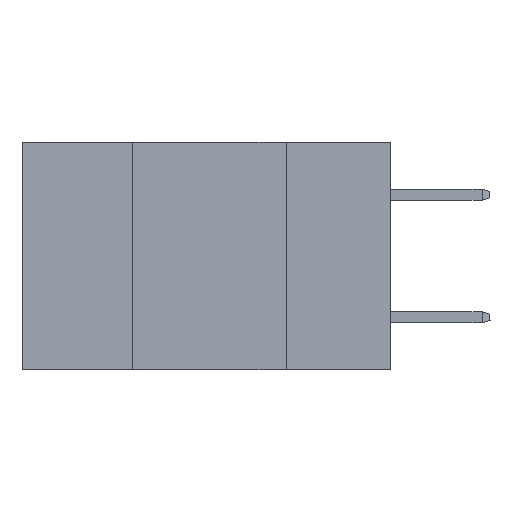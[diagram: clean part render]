
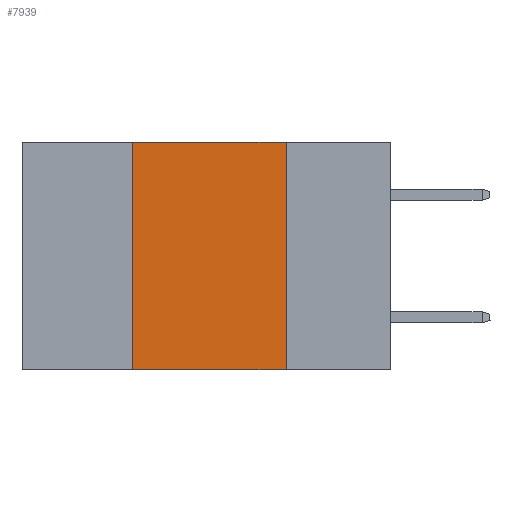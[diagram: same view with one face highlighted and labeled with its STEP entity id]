
A CAD part, left-side view. The second image highlights one B-rep face of the part: STEP entity #7939.
In plain terms, the highlighted planar face has unit normal (-1, 0, 0).
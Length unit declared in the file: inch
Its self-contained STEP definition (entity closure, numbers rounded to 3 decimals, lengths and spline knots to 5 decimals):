
#281 = LINE ( 'NONE', #3648, #5363 ) ;
#696 = EDGE_CURVE ( 'NONE', #11464, #17121, #1826, .T. ) ;
#832 = EDGE_LOOP ( 'NONE', ( #17126, #20765, #9822, #13039 ) ) ;
#1763 = DIRECTION ( 'NONE',  ( 0., 0., 1. ) ) ;
#1826 = LINE ( 'NONE', #14221, #5634 ) ;
#2089 = DIRECTION ( 'NONE',  ( 0., 0., -1. ) ) ;
#2645 = CARTESIAN_POINT ( 'NONE',  ( 0., 0.17, 0. ) ) ;
#3424 = EDGE_CURVE ( 'NONE', #17121, #15181, #281, .T. ) ;
#3464 = CARTESIAN_POINT ( 'NONE',  ( 0., 0.42, 0. ) ) ;
#3470 = CARTESIAN_POINT ( 'NONE',  ( 0., 0.6, 0. ) ) ;
#3648 = CARTESIAN_POINT ( 'NONE',  ( 0., 0.17, 0. ) ) ;
#5363 = VECTOR ( 'NONE', #2089, 39.37008 ) ;
#5634 = VECTOR ( 'NONE', #9278, 39.37008 ) ;
#6985 = PLANE ( 'NONE',  #19866 ) ;
#7691 = CARTESIAN_POINT ( 'NONE',  ( 0., 0.6, -0.37 ) ) ;
#7939 = ADVANCED_FACE ( 'NONE', ( #20541 ), #6985, .F. ) ;
#8173 = CARTESIAN_POINT ( 'NONE',  ( 0., 0.17, -0.37 ) ) ;
#8841 = VECTOR ( 'NONE', #1763, 39.37008 ) ;
#9220 = DIRECTION ( 'NONE',  ( 0., -1., 0. ) ) ;
#9278 = DIRECTION ( 'NONE',  ( 0., -1., 0. ) ) ;
#9508 = EDGE_CURVE ( 'NONE', #11034, #15181, #20712, .T. ) ;
#9822 = ORIENTED_EDGE ( 'NONE', *, *, #20562, .F. ) ;
#10259 = DIRECTION ( 'NONE',  ( 0., 0., -1. ) ) ;
#10483 = CARTESIAN_POINT ( 'NONE',  ( 0., 0.42, -0.37 ) ) ;
#11034 = VERTEX_POINT ( 'NONE', #10483 ) ;
#11436 = DIRECTION ( 'NONE',  ( 1., 0., 0. ) ) ;
#11464 = VERTEX_POINT ( 'NONE', #20120 ) ;
#13039 = ORIENTED_EDGE ( 'NONE', *, *, #9508, .T. ) ;
#13930 = VECTOR ( 'NONE', #9220, 39.37008 ) ;
#14221 = CARTESIAN_POINT ( 'NONE',  ( 0., 0.6, 0. ) ) ;
#15181 = VERTEX_POINT ( 'NONE', #8173 ) ;
#17121 = VERTEX_POINT ( 'NONE', #2645 ) ;
#17126 = ORIENTED_EDGE ( 'NONE', *, *, #3424, .F. ) ;
#17413 = LINE ( 'NONE', #3464, #8841 ) ;
#19866 = AXIS2_PLACEMENT_3D ( 'NONE', #3470, #11436, #10259 ) ;
#20120 = CARTESIAN_POINT ( 'NONE',  ( 0., 0.42, 0. ) ) ;
#20541 = FACE_OUTER_BOUND ( 'NONE', #832, .T. ) ;
#20562 = EDGE_CURVE ( 'NONE', #11034, #11464, #17413, .T. ) ;
#20712 = LINE ( 'NONE', #7691, #13930 ) ;
#20765 = ORIENTED_EDGE ( 'NONE', *, *, #696, .F. ) ;
